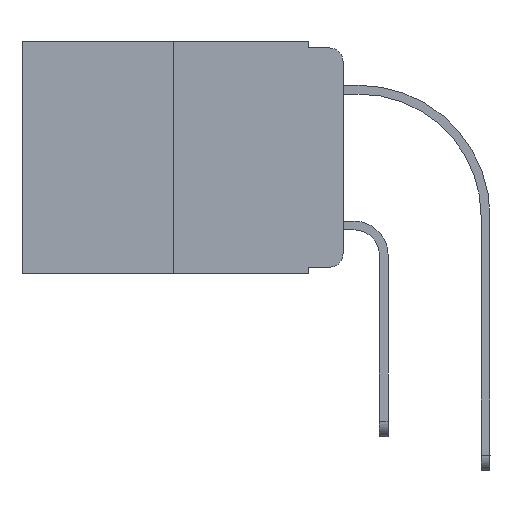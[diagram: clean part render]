
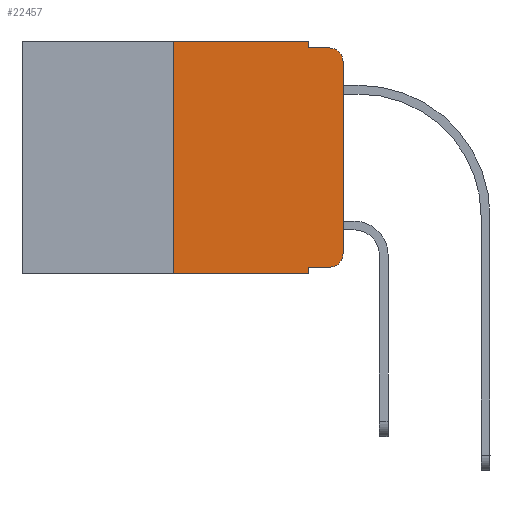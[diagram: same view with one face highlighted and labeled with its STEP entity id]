
A CAD part, left-side view. The second image highlights one B-rep face of the part: STEP entity #22457.
In plain terms, the highlighted planar face has unit normal (-1, 0, 0).
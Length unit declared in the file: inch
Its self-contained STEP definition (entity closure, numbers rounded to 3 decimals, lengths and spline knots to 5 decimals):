
#397 = DIRECTION ( 'NONE',  ( 0., 0., -1. ) ) ;
#408 = AXIS2_PLACEMENT_3D ( 'NONE', #4147, #11525, #397 ) ;
#912 = LINE ( 'NONE', #10343, #9218 ) ;
#1045 = AXIS2_PLACEMENT_3D ( 'NONE', #15990, #23470, #19834 ) ;
#1212 = DIRECTION ( 'NONE',  ( 0., -1., 0. ) ) ;
#1409 = DIRECTION ( 'NONE',  ( 0., 0., -1. ) ) ;
#1602 = DIRECTION ( 'NONE',  ( 0., -1., 0. ) ) ;
#1633 = VECTOR ( 'NONE', #14098, 39.37008 ) ;
#1841 = EDGE_CURVE ( 'NONE', #7551, #17467, #19193, .T. ) ;
#1871 = EDGE_CURVE ( 'NONE', #4332, #10882, #17737, .T. ) ;
#1914 = CARTESIAN_POINT ( 'NONE',  ( 0., 0., -0.313 ) ) ;
#2754 = LINE ( 'NONE', #12186, #10266 ) ;
#2849 = CARTESIAN_POINT ( 'NONE',  ( 0., 0., -0.03 ) ) ;
#2858 = VERTEX_POINT ( 'NONE', #2849 ) ;
#4147 = CARTESIAN_POINT ( 'NONE',  ( 0., 0.02, -0.313 ) ) ;
#4332 = VERTEX_POINT ( 'NONE', #9032 ) ;
#5288 = CARTESIAN_POINT ( 'NONE',  ( 0., 0.25, 0. ) ) ;
#6564 = DIRECTION ( 'NONE',  ( 0., 0., -1. ) ) ;
#6835 = CARTESIAN_POINT ( 'NONE',  ( 0., 0.051, 0. ) ) ;
#7124 = LINE ( 'NONE', #16593, #20808 ) ;
#7222 = EDGE_CURVE ( 'NONE', #15975, #10882, #16671, .T. ) ;
#7429 = EDGE_CURVE ( 'NONE', #15975, #15886, #912, .T. ) ;
#7551 = VERTEX_POINT ( 'NONE', #19206 ) ;
#7556 = VERTEX_POINT ( 'NONE', #9984 ) ;
#8096 = ORIENTED_EDGE ( 'NONE', *, *, #15238, .F. ) ;
#8254 = CIRCLE ( 'NONE', #17944, 0.02 ) ;
#8487 = DIRECTION ( 'NONE',  ( -1., 0., 0. ) ) ;
#9017 = CARTESIAN_POINT ( 'NONE',  ( 0., 0.051, 0. ) ) ;
#9032 = CARTESIAN_POINT ( 'NONE',  ( 0., 0.25, -0.343 ) ) ;
#9218 = VECTOR ( 'NONE', #17750, 39.37008 ) ;
#9984 = CARTESIAN_POINT ( 'NONE',  ( 0., 0.051, -0.01 ) ) ;
#10266 = VECTOR ( 'NONE', #17300, 39.37008 ) ;
#10343 = CARTESIAN_POINT ( 'NONE',  ( 0., 0.051, -0.333 ) ) ;
#10801 = CARTESIAN_POINT ( 'NONE',  ( 0., 0.473, 0. ) ) ;
#10882 = VERTEX_POINT ( 'NONE', #13500 ) ;
#11455 = CARTESIAN_POINT ( 'NONE',  ( 0., 0.02, -0.333 ) ) ;
#11525 = DIRECTION ( 'NONE',  ( -1., 0., 0. ) ) ;
#12044 = ORIENTED_EDGE ( 'NONE', *, *, #21003, .F. ) ;
#12186 = CARTESIAN_POINT ( 'NONE',  ( 0., 0.051, 0. ) ) ;
#12247 = CARTESIAN_POINT ( 'NONE',  ( 0., 0.02, -0.03 ) ) ;
#12320 = ORIENTED_EDGE ( 'NONE', *, *, #1871, .T. ) ;
#12334 = VECTOR ( 'NONE', #14742, 39.37008 ) ;
#12440 = FACE_OUTER_BOUND ( 'NONE', #12762, .T. ) ;
#12762 = EDGE_LOOP ( 'NONE', ( #22831, #13655, #8096, #12044, #23628, #19736, #12320, #17183, #17424, #19080 ) ) ;
#13500 = CARTESIAN_POINT ( 'NONE',  ( 0., 0.051, -0.343 ) ) ;
#13655 = ORIENTED_EDGE ( 'NONE', *, *, #23775, .T. ) ;
#14098 = DIRECTION ( 'NONE',  ( 0., -1., 0. ) ) ;
#14440 = CARTESIAN_POINT ( 'NONE',  ( 0., 0.473, -0.343 ) ) ;
#14742 = DIRECTION ( 'NONE',  ( 0., 0., 1. ) ) ;
#15019 = VECTOR ( 'NONE', #1409, 39.37008 ) ;
#15238 = EDGE_CURVE ( 'NONE', #7556, #21403, #19616, .T. ) ;
#15364 = EDGE_CURVE ( 'NONE', #20800, #2858, #7124, .T. ) ;
#15493 = CIRCLE ( 'NONE', #408, 0.02 ) ;
#15886 = VERTEX_POINT ( 'NONE', #11455 ) ;
#15975 = VERTEX_POINT ( 'NONE', #21377 ) ;
#15990 = CARTESIAN_POINT ( 'NONE',  ( 0., 0.473, 0. ) ) ;
#16110 = PLANE ( 'NONE',  #1045 ) ;
#16593 = CARTESIAN_POINT ( 'NONE',  ( 0., 0., 0. ) ) ;
#16671 = LINE ( 'NONE', #9017, #15019 ) ;
#17109 = EDGE_CURVE ( 'NONE', #4332, #7551, #21885, .T. ) ;
#17183 = ORIENTED_EDGE ( 'NONE', *, *, #7222, .F. ) ;
#17300 = DIRECTION ( 'NONE',  ( 0., 0., -1. ) ) ;
#17424 = ORIENTED_EDGE ( 'NONE', *, *, #7429, .T. ) ;
#17467 = VERTEX_POINT ( 'NONE', #6835 ) ;
#17500 = CARTESIAN_POINT ( 'NONE',  ( 0., 0.02, -0.01 ) ) ;
#17501 = VECTOR ( 'NONE', #1602, 39.37008 ) ;
#17737 = LINE ( 'NONE', #14440, #17501 ) ;
#17750 = DIRECTION ( 'NONE',  ( 0., -1., 0. ) ) ;
#17944 = AXIS2_PLACEMENT_3D ( 'NONE', #12247, #8487, #6564 ) ;
#18037 = DIRECTION ( 'NONE',  ( 0., 0., 1. ) ) ;
#18140 = EDGE_CURVE ( 'NONE', #15886, #20800, #15493, .T. ) ;
#19080 = ORIENTED_EDGE ( 'NONE', *, *, #18140, .T. ) ;
#19193 = LINE ( 'NONE', #10801, #1633 ) ;
#19206 = CARTESIAN_POINT ( 'NONE',  ( 0., 0.25, 0. ) ) ;
#19266 = CARTESIAN_POINT ( 'NONE',  ( 0., 0.051, -0.01 ) ) ;
#19616 = LINE ( 'NONE', #19266, #22353 ) ;
#19736 = ORIENTED_EDGE ( 'NONE', *, *, #17109, .F. ) ;
#19834 = DIRECTION ( 'NONE',  ( 0., 0., -1. ) ) ;
#20800 = VERTEX_POINT ( 'NONE', #1914 ) ;
#20808 = VECTOR ( 'NONE', #18037, 39.37008 ) ;
#21003 = EDGE_CURVE ( 'NONE', #17467, #7556, #2754, .T. ) ;
#21377 = CARTESIAN_POINT ( 'NONE',  ( 0., 0.051, -0.333 ) ) ;
#21403 = VERTEX_POINT ( 'NONE', #17500 ) ;
#21885 = LINE ( 'NONE', #5288, #12334 ) ;
#22353 = VECTOR ( 'NONE', #1212, 39.37008 ) ;
#22457 = ADVANCED_FACE ( 'NONE', ( #12440 ), #16110, .F. ) ;
#22831 = ORIENTED_EDGE ( 'NONE', *, *, #15364, .T. ) ;
#23470 = DIRECTION ( 'NONE',  ( 1., 0., 0. ) ) ;
#23628 = ORIENTED_EDGE ( 'NONE', *, *, #1841, .F. ) ;
#23775 = EDGE_CURVE ( 'NONE', #2858, #21403, #8254, .T. ) ;
